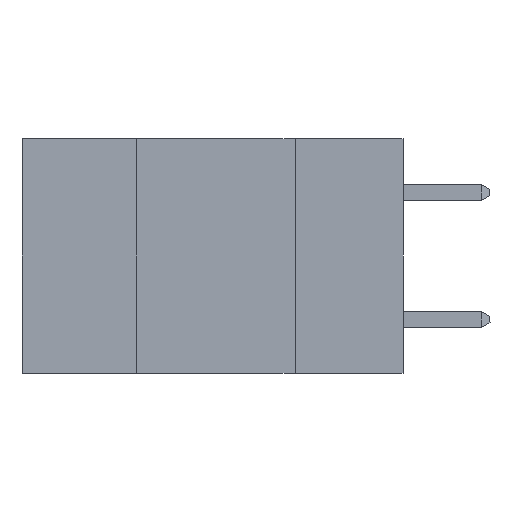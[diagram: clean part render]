
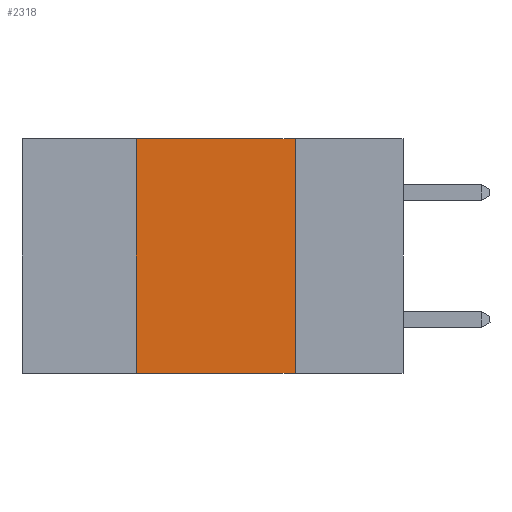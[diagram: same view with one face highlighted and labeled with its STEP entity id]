
A CAD part, left-side view. The second image highlights one B-rep face of the part: STEP entity #2318.
In plain terms, the highlighted planar face has unit normal (-1, 0, 0).
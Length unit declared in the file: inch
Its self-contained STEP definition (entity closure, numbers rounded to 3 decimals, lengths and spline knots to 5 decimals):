
#46 = DIRECTION ( 'NONE',  ( 0., -1., 0. ) ) ;
#999 = EDGE_CURVE ( 'NONE', #7736, #9535, #14361, .T. ) ;
#1524 = CARTESIAN_POINT ( 'NONE',  ( 0., 0.6, 0. ) ) ;
#2318 = ADVANCED_FACE ( 'NONE', ( #11672 ), #10063, .F. ) ;
#2754 = CARTESIAN_POINT ( 'NONE',  ( 0., 0.42, 0. ) ) ;
#5719 = ORIENTED_EDGE ( 'NONE', *, *, #999, .F. ) ;
#6773 = DIRECTION ( 'NONE',  ( 0., 0., -1. ) ) ;
#6858 = CARTESIAN_POINT ( 'NONE',  ( 0., 0.17, 0. ) ) ;
#7611 = EDGE_LOOP ( 'NONE', ( #5719, #15787, #17667, #14487 ) ) ;
#7736 = VERTEX_POINT ( 'NONE', #14129 ) ;
#8420 = VECTOR ( 'NONE', #46, 39.37008 ) ;
#8855 = AXIS2_PLACEMENT_3D ( 'NONE', #9965, #9941, #9907 ) ;
#9313 = CARTESIAN_POINT ( 'NONE',  ( 0., 0.42, -0.37 ) ) ;
#9448 = CARTESIAN_POINT ( 'NONE',  ( 0., 0.17, -0.37 ) ) ;
#9535 = VERTEX_POINT ( 'NONE', #9448 ) ;
#9907 = DIRECTION ( 'NONE',  ( 0., 0., -1. ) ) ;
#9941 = DIRECTION ( 'NONE',  ( 1., 0., 0. ) ) ;
#9965 = CARTESIAN_POINT ( 'NONE',  ( 0., 0.6, 0. ) ) ;
#10063 = PLANE ( 'NONE',  #8855 ) ;
#11672 = FACE_OUTER_BOUND ( 'NONE', #7611, .T. ) ;
#12112 = LINE ( 'NONE', #1524, #8420 ) ;
#12307 = VECTOR ( 'NONE', #15856, 39.37008 ) ;
#13844 = DIRECTION ( 'NONE',  ( 0., -1., 0. ) ) ;
#14040 = VERTEX_POINT ( 'NONE', #2754 ) ;
#14129 = CARTESIAN_POINT ( 'NONE',  ( 0., 0.17, 0. ) ) ;
#14361 = LINE ( 'NONE', #6858, #17070 ) ;
#14445 = VERTEX_POINT ( 'NONE', #9313 ) ;
#14487 = ORIENTED_EDGE ( 'NONE', *, *, #15745, .T. ) ;
#14831 = LINE ( 'NONE', #15179, #17559 ) ;
#15179 = CARTESIAN_POINT ( 'NONE',  ( 0., 0.6, -0.37 ) ) ;
#15192 = EDGE_CURVE ( 'NONE', #14040, #7736, #12112, .T. ) ;
#15402 = EDGE_CURVE ( 'NONE', #14445, #14040, #15909, .T. ) ;
#15745 = EDGE_CURVE ( 'NONE', #14445, #9535, #14831, .T. ) ;
#15787 = ORIENTED_EDGE ( 'NONE', *, *, #15192, .F. ) ;
#15856 = DIRECTION ( 'NONE',  ( 0., 0., 1. ) ) ;
#15909 = LINE ( 'NONE', #17129, #12307 ) ;
#17070 = VECTOR ( 'NONE', #6773, 39.37008 ) ;
#17129 = CARTESIAN_POINT ( 'NONE',  ( 0., 0.42, 0. ) ) ;
#17559 = VECTOR ( 'NONE', #13844, 39.37008 ) ;
#17667 = ORIENTED_EDGE ( 'NONE', *, *, #15402, .F. ) ;
